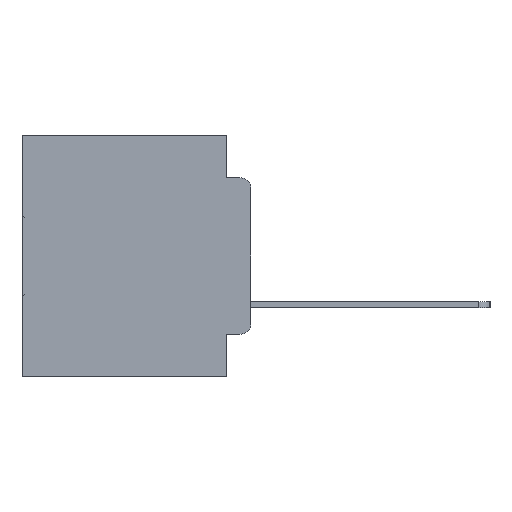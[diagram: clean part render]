
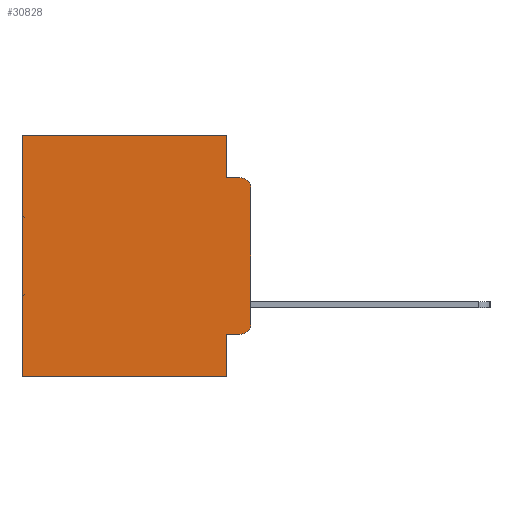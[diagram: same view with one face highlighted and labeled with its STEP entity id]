
A CAD part, left-side view. The second image highlights one B-rep face of the part: STEP entity #30828.
In plain terms, the highlighted planar face has unit normal (-1, 0, 0).
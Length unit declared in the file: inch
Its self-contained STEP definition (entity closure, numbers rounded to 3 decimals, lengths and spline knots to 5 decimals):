
#594 = VERTEX_POINT ( 'NONE', #6890 ) ;
#1449 = VECTOR ( 'NONE', #32651, 39.37008 ) ;
#1624 = ORIENTED_EDGE ( 'NONE', *, *, #20888, .T. ) ;
#2341 = DIRECTION ( 'NONE',  ( -1., 0., 0. ) ) ;
#4542 = LINE ( 'NONE', #20475, #17886 ) ;
#4689 = VERTEX_POINT ( 'NONE', #21109 ) ;
#5096 = EDGE_CURVE ( 'NONE', #27287, #25660, #8832, .T. ) ;
#6254 = CARTESIAN_POINT ( 'NONE',  ( 0.298, 0., 0. ) ) ;
#6766 = LINE ( 'NONE', #14106, #32813 ) ;
#6798 = VECTOR ( 'NONE', #29789, 39.37008 ) ;
#6890 = CARTESIAN_POINT ( 'NONE',  ( 0.298, 0., -0.3915 ) ) ;
#7411 = VERTEX_POINT ( 'NONE', #7539 ) ;
#7539 = CARTESIAN_POINT ( 'NONE',  ( 0.298, 0.051, -0.5 ) ) ;
#7910 = FACE_OUTER_BOUND ( 'NONE', #20843, .T. ) ;
#8091 = ORIENTED_EDGE ( 'NONE', *, *, #32616, .T. ) ;
#8646 = EDGE_CURVE ( 'NONE', #10471, #32149, #25207, .T. ) ;
#8671 = ORIENTED_EDGE ( 'NONE', *, *, #5096, .T. ) ;
#8832 = LINE ( 'NONE', #30080, #1449 ) ;
#8995 = DIRECTION ( 'NONE',  ( 1., 0., 0. ) ) ;
#9320 = EDGE_CURVE ( 'NONE', #4689, #594, #30952, .T. ) ;
#9345 = ORIENTED_EDGE ( 'NONE', *, *, #21317, .F. ) ;
#9650 = EDGE_CURVE ( 'NONE', #7411, #22496, #4542, .T. ) ;
#10117 = ORIENTED_EDGE ( 'NONE', *, *, #17467, .F. ) ;
#10167 = DIRECTION ( 'NONE',  ( 0., 1., 0. ) ) ;
#10471 = VERTEX_POINT ( 'NONE', #19752 ) ;
#10486 = CARTESIAN_POINT ( 'NONE',  ( 0.298, 0.02, -0.4115 ) ) ;
#11585 = CARTESIAN_POINT ( 'NONE',  ( 0.298, 0.051, 0. ) ) ;
#12425 = VECTOR ( 'NONE', #14252, 39.37008 ) ;
#12778 = ORIENTED_EDGE ( 'NONE', *, *, #9320, .F. ) ;
#13531 = CARTESIAN_POINT ( 'NONE',  ( 0.298, 0.02, -0.1085 ) ) ;
#14066 = DIRECTION ( 'NONE',  ( 0., -1., 0. ) ) ;
#14106 = CARTESIAN_POINT ( 'NONE',  ( 0.298, 0.051, 0. ) ) ;
#14252 = DIRECTION ( 'NONE',  ( 0., 0., -1. ) ) ;
#14941 = CARTESIAN_POINT ( 'NONE',  ( 0.298, 0.473, 0. ) ) ;
#16012 = VERTEX_POINT ( 'NONE', #10486 ) ;
#16149 = DIRECTION ( 'NONE',  ( 0., 0., -1. ) ) ;
#16479 = DIRECTION ( 'NONE',  ( 0., 0., -1. ) ) ;
#16522 = DIRECTION ( 'NONE',  ( 0., -1., 0. ) ) ;
#16547 = CARTESIAN_POINT ( 'NONE',  ( 0.298, 0.051, -0.4115 ) ) ;
#16825 = CIRCLE ( 'NONE', #31466, 0.02 ) ;
#17428 = CARTESIAN_POINT ( 'NONE',  ( 0.298, 0.473, 0. ) ) ;
#17467 = EDGE_CURVE ( 'NONE', #27287, #10471, #19323, .T. ) ;
#17886 = VECTOR ( 'NONE', #10167, 39.37008 ) ;
#18423 = CARTESIAN_POINT ( 'NONE',  ( 0.298, 0.02, -0.3915 ) ) ;
#18667 = VECTOR ( 'NONE', #16522, 39.37008 ) ;
#19323 = LINE ( 'NONE', #11585, #12425 ) ;
#19752 = CARTESIAN_POINT ( 'NONE',  ( 0.298, 0.051, -0.0885 ) ) ;
#20164 = CARTESIAN_POINT ( 'NONE',  ( 0.298, 0.473, -0.5 ) ) ;
#20475 = CARTESIAN_POINT ( 'NONE',  ( 0.298, 0., -0.5 ) ) ;
#20628 = VECTOR ( 'NONE', #14066, 39.37008 ) ;
#20843 = EDGE_LOOP ( 'NONE', ( #12778, #30514, #22230, #10117, #8671, #1624, #30620, #9345, #23835, #8091 ) ) ;
#20888 = EDGE_CURVE ( 'NONE', #25660, #22496, #32839, .T. ) ;
#20935 = DIRECTION ( 'NONE',  ( 0., 0., -1. ) ) ;
#21109 = CARTESIAN_POINT ( 'NONE',  ( 0.298, 0., -0.1085 ) ) ;
#21317 = EDGE_CURVE ( 'NONE', #26238, #7411, #6766, .T. ) ;
#22188 = LINE ( 'NONE', #16547, #20628 ) ;
#22230 = ORIENTED_EDGE ( 'NONE', *, *, #8646, .F. ) ;
#22496 = VERTEX_POINT ( 'NONE', #20164 ) ;
#22950 = EDGE_CURVE ( 'NONE', #26238, #16012, #22188, .T. ) ;
#23835 = ORIENTED_EDGE ( 'NONE', *, *, #22950, .T. ) ;
#24273 = DIRECTION ( 'NONE',  ( 0., 0., -1. ) ) ;
#24378 = PLANE ( 'NONE',  #31034 ) ;
#24379 = CARTESIAN_POINT ( 'NONE',  ( 0.298, 0.02, -0.0885 ) ) ;
#25207 = LINE ( 'NONE', #26402, #18667 ) ;
#25300 = VECTOR ( 'NONE', #16479, 39.37008 ) ;
#25660 = VERTEX_POINT ( 'NONE', #17428 ) ;
#26238 = VERTEX_POINT ( 'NONE', #26698 ) ;
#26402 = CARTESIAN_POINT ( 'NONE',  ( 0.298, 0.051, -0.0885 ) ) ;
#26549 = CARTESIAN_POINT ( 'NONE',  ( 0.298, 0.051, 0. ) ) ;
#26698 = CARTESIAN_POINT ( 'NONE',  ( 0.298, 0.051, -0.4115 ) ) ;
#26797 = DIRECTION ( 'NONE',  ( 0., 0., -1. ) ) ;
#27287 = VERTEX_POINT ( 'NONE', #26549 ) ;
#28309 = CIRCLE ( 'NONE', #31789, 0.02 ) ;
#29632 = EDGE_CURVE ( 'NONE', #4689, #32149, #28309, .T. ) ;
#29789 = DIRECTION ( 'NONE',  ( 0., 0., -1. ) ) ;
#30080 = CARTESIAN_POINT ( 'NONE',  ( 0.298, 0., 0. ) ) ;
#30514 = ORIENTED_EDGE ( 'NONE', *, *, #29632, .T. ) ;
#30620 = ORIENTED_EDGE ( 'NONE', *, *, #9650, .F. ) ;
#30828 = ADVANCED_FACE ( 'NONE', ( #7910 ), #24378, .F. ) ;
#30894 = DIRECTION ( 'NONE',  ( -1., 0., 0. ) ) ;
#30952 = LINE ( 'NONE', #31205, #25300 ) ;
#31034 = AXIS2_PLACEMENT_3D ( 'NONE', #6254, #8995, #26797 ) ;
#31205 = CARTESIAN_POINT ( 'NONE',  ( 0.298, 0., 0. ) ) ;
#31466 = AXIS2_PLACEMENT_3D ( 'NONE', #18423, #2341, #20935 ) ;
#31789 = AXIS2_PLACEMENT_3D ( 'NONE', #13531, #30894, #16149 ) ;
#32149 = VERTEX_POINT ( 'NONE', #24379 ) ;
#32616 = EDGE_CURVE ( 'NONE', #16012, #594, #16825, .T. ) ;
#32651 = DIRECTION ( 'NONE',  ( 0., 1., 0. ) ) ;
#32813 = VECTOR ( 'NONE', #24273, 39.37008 ) ;
#32839 = LINE ( 'NONE', #14941, #6798 ) ;
